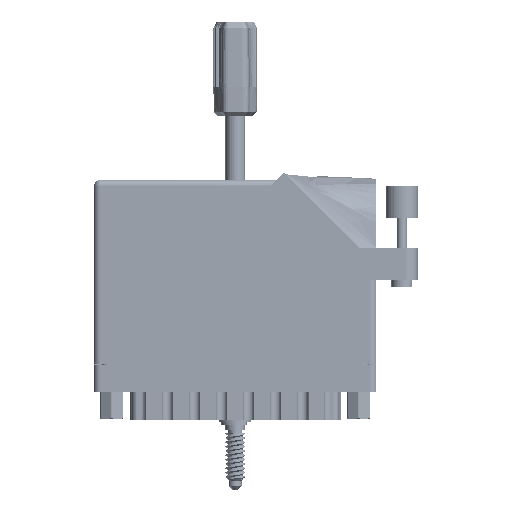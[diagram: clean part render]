
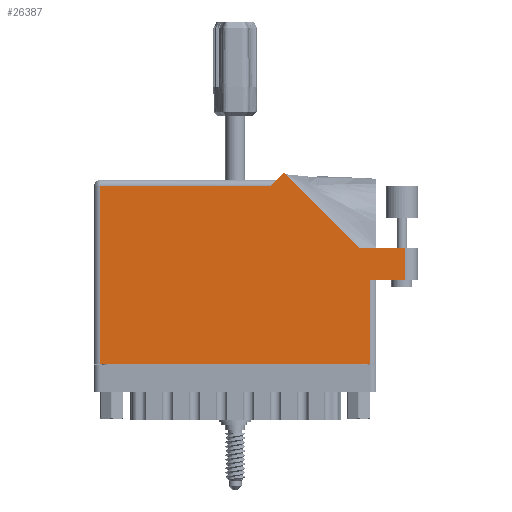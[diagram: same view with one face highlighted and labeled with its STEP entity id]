
A CAD part, front view. The second image highlights one B-rep face of the part: STEP entity #26387.
In plain terms, the highlighted face is planar.
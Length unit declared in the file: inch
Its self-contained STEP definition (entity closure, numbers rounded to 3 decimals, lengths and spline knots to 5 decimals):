
#102 = LINE ( 'NONE', #15975, #56353 ) ;
#205 = VERTEX_POINT ( 'NONE', #64557 ) ;
#6146 = ORIENTED_EDGE ( 'NONE', *, *, #36095, .T. ) ;
#9672 = LINE ( 'NONE', #76923, #10927 ) ;
#10927 = VECTOR ( 'NONE', #31222, 39.37008 ) ;
#12887 = CARTESIAN_POINT ( 'NONE',  ( 2.55242, 1.122, 0. ) ) ;
#13046 = VECTOR ( 'NONE', #65793, 39.37008 ) ;
#14673 = EDGE_LOOP ( 'NONE', ( #68560, #6146, #67788, #30303, #61432, #52102, #56304, #28324, #54938 ) ) ;
#15975 = CARTESIAN_POINT ( 'NONE',  ( 2.718, 0.815, 0. ) ) ;
#17198 = CARTESIAN_POINT ( 'NONE',  ( 1.758, 1.775, 0. ) ) ;
#17347 = EDGE_CURVE ( 'NONE', #57578, #39171, #33587, .T. ) ;
#18410 = PLANE ( 'NONE',  #80656 ) ;
#20655 = VECTOR ( 'NONE', #46997, 39.37008 ) ;
#21458 = LINE ( 'NONE', #77058, #59780 ) ;
#22995 = DIRECTION ( 'NONE',  ( 1., 0., 0. ) ) ;
#26387 = ADVANCED_FACE ( 'NONE', ( #37822 ), #18410, .F. ) ;
#28323 = VERTEX_POINT ( 'NONE', #98182 ) ;
#28324 = ORIENTED_EDGE ( 'NONE', *, *, #81554, .T. ) ;
#30303 = ORIENTED_EDGE ( 'NONE', *, *, #42818, .T. ) ;
#30438 = LINE ( 'NONE', #64826, #48364 ) ;
#30920 = EDGE_CURVE ( 'NONE', #93393, #33676, #89422, .T. ) ;
#31222 = DIRECTION ( 'NONE',  ( 0., 1., 0. ) ) ;
#32441 = CARTESIAN_POINT ( 'NONE',  ( 0., 0., 0. ) ) ;
#33587 = LINE ( 'NONE', #17198, #87299 ) ;
#33676 = VERTEX_POINT ( 'NONE', #84263 ) ;
#33758 = DIRECTION ( 'NONE',  ( 1., 0., 0. ) ) ;
#33838 = CARTESIAN_POINT ( 'NONE',  ( 0., 1.775, 0. ) ) ;
#36095 = EDGE_CURVE ( 'NONE', #61094, #205, #9672, .T. ) ;
#36913 = EDGE_CURVE ( 'NONE', #33676, #61094, #102, .T. ) ;
#37822 = FACE_OUTER_BOUND ( 'NONE', #14673, .T. ) ;
#38645 = LINE ( 'NONE', #78003, #20655 ) ;
#39171 = VERTEX_POINT ( 'NONE', #97386 ) ;
#39613 = LINE ( 'NONE', #32441, #65878 ) ;
#42818 = EDGE_CURVE ( 'NONE', #55417, #57578, #21458, .T. ) ;
#46997 = DIRECTION ( 'NONE',  ( -1., 0., 0. ) ) ;
#48364 = VECTOR ( 'NONE', #79143, 39.37008 ) ;
#52102 = ORIENTED_EDGE ( 'NONE', *, *, #90400, .T. ) ;
#52313 = CARTESIAN_POINT ( 'NONE',  ( 1.82871, 1.84571, 0. ) ) ;
#54938 = ORIENTED_EDGE ( 'NONE', *, *, #30920, .T. ) ;
#55417 = VERTEX_POINT ( 'NONE', #12887 ) ;
#55625 = EDGE_CURVE ( 'NONE', #205, #55417, #38645, .T. ) ;
#56304 = ORIENTED_EDGE ( 'NONE', *, *, #98441, .T. ) ;
#56353 = VECTOR ( 'NONE', #22995, 39.37008 ) ;
#57578 = VERTEX_POINT ( 'NONE', #52313 ) ;
#58111 = CARTESIAN_POINT ( 'NONE',  ( 0.062, 0., 0. ) ) ;
#58384 = CARTESIAN_POINT ( 'NONE',  ( 2.656, 0., 0. ) ) ;
#59780 = VECTOR ( 'NONE', #92708, 39.37008 ) ;
#61094 = VERTEX_POINT ( 'NONE', #65210 ) ;
#61432 = ORIENTED_EDGE ( 'NONE', *, *, #17347, .T. ) ;
#64371 = VECTOR ( 'NONE', #76771, 39.37008 ) ;
#64557 = CARTESIAN_POINT ( 'NONE',  ( 2.993, 1.122, 0. ) ) ;
#64826 = CARTESIAN_POINT ( 'NONE',  ( 0., 1.713, 0. ) ) ;
#65210 = CARTESIAN_POINT ( 'NONE',  ( 2.993, 0.815, 0. ) ) ;
#65793 = DIRECTION ( 'NONE',  ( 0., -1., 0. ) ) ;
#65878 = VECTOR ( 'NONE', #33758, 39.37008 ) ;
#67788 = ORIENTED_EDGE ( 'NONE', *, *, #55625, .T. ) ;
#68560 = ORIENTED_EDGE ( 'NONE', *, *, #36913, .T. ) ;
#71025 = DIRECTION ( 'NONE',  ( -0.707, -0.707, 0. ) ) ;
#76771 = DIRECTION ( 'NONE',  ( 0., 1., 0. ) ) ;
#76923 = CARTESIAN_POINT ( 'NONE',  ( 2.993, 1.122, 0. ) ) ;
#77058 = CARTESIAN_POINT ( 'NONE',  ( 2.55242, 1.122, 0. ) ) ;
#77665 = VERTEX_POINT ( 'NONE', #89446 ) ;
#78003 = CARTESIAN_POINT ( 'NONE',  ( 3.118, 1.122, 0. ) ) ;
#79143 = DIRECTION ( 'NONE',  ( -1., 0., 0. ) ) ;
#80656 = AXIS2_PLACEMENT_3D ( 'NONE', #33838, #87232, #87558 ) ;
#81554 = EDGE_CURVE ( 'NONE', #28323, #93393, #39613, .T. ) ;
#83620 = LINE ( 'NONE', #58111, #13046 ) ;
#84263 = CARTESIAN_POINT ( 'NONE',  ( 2.656, 0.815, 0. ) ) ;
#87232 = DIRECTION ( 'NONE',  ( 0., 0., -1. ) ) ;
#87299 = VECTOR ( 'NONE', #71025, 39.37008 ) ;
#87558 = DIRECTION ( 'NONE',  ( -1., 0., 0. ) ) ;
#89422 = LINE ( 'NONE', #92434, #64371 ) ;
#89446 = CARTESIAN_POINT ( 'NONE',  ( 0.062, 1.713, 0. ) ) ;
#90400 = EDGE_CURVE ( 'NONE', #39171, #77665, #30438, .T. ) ;
#92434 = CARTESIAN_POINT ( 'NONE',  ( 2.656, 0.815, 0. ) ) ;
#92708 = DIRECTION ( 'NONE',  ( -0.707, 0.707, 0. ) ) ;
#93393 = VERTEX_POINT ( 'NONE', #58384 ) ;
#97386 = CARTESIAN_POINT ( 'NONE',  ( 1.696, 1.713, 0. ) ) ;
#98182 = CARTESIAN_POINT ( 'NONE',  ( 0.062, 0., 0. ) ) ;
#98441 = EDGE_CURVE ( 'NONE', #77665, #28323, #83620, .T. ) ;
